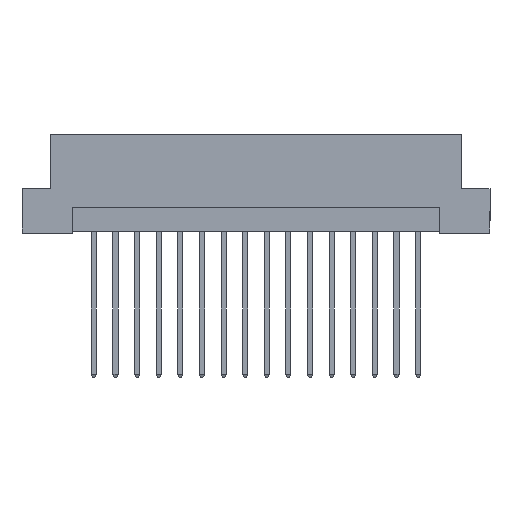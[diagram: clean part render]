
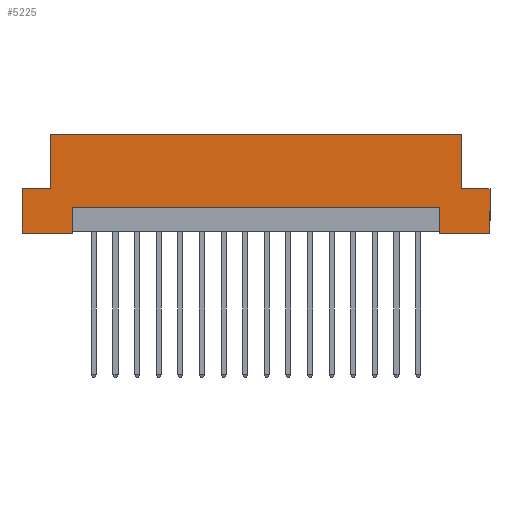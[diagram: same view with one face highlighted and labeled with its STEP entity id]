
A CAD part, front view. The second image highlights one B-rep face of the part: STEP entity #5225.
In plain terms, the highlighted planar face has unit normal (0, -1, 0).
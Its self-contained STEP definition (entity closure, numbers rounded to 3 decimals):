
#166 = ORIENTED_EDGE ( 'NONE', *, *, #7190, .F. ) ;
#254 = EDGE_CURVE ( 'NONE', #5056, #949, #5466, .T. ) ;
#280 = FACE_OUTER_BOUND ( 'NONE', #7388, .T. ) ;
#286 = CARTESIAN_POINT ( 'NONE',  ( 21.6, -4.3, 0.2 ) ) ;
#355 = DIRECTION ( 'NONE',  ( 1., 0., 0. ) ) ;
#407 = ORIENTED_EDGE ( 'NONE', *, *, #4334, .F. ) ;
#423 = EDGE_CURVE ( 'NONE', #5056, #5381, #3980, .T. ) ;
#424 = DIRECTION ( 'NONE',  ( 1., 0., 0. ) ) ;
#456 = CARTESIAN_POINT ( 'NONE',  ( -21.6, -4.3, 0.2 ) ) ;
#461 = DIRECTION ( 'NONE',  ( 1., 0., 0. ) ) ;
#501 = CARTESIAN_POINT ( 'NONE',  ( -24.2, -4.3, 11.6 ) ) ;
#583 = CARTESIAN_POINT ( 'NONE',  ( -27.5, -4.3, 5.2 ) ) ;
#593 = CARTESIAN_POINT ( 'NONE',  ( 21.6, -4.3, 3. ) ) ;
#705 = CARTESIAN_POINT ( 'NONE',  ( 27.5, -4.3, 11.6 ) ) ;
#861 = ORIENTED_EDGE ( 'NONE', *, *, #946, .F. ) ;
#903 = CARTESIAN_POINT ( 'NONE',  ( 24.2, -4.3, 5.2 ) ) ;
#932 = LINE ( 'NONE', #286, #4435 ) ;
#946 = EDGE_CURVE ( 'NONE', #5382, #5692, #3523, .T. ) ;
#949 = VERTEX_POINT ( 'NONE', #593 ) ;
#1036 = VECTOR ( 'NONE', #1269, 1000. ) ;
#1092 = ORIENTED_EDGE ( 'NONE', *, *, #1218, .F. ) ;
#1218 = EDGE_CURVE ( 'NONE', #6092, #949, #932, .T. ) ;
#1231 = ORIENTED_EDGE ( 'NONE', *, *, #1559, .F. ) ;
#1269 = DIRECTION ( 'NONE',  ( 0., 0., -1. ) ) ;
#1309 = CARTESIAN_POINT ( 'NONE',  ( -24.2, -4.3, 5.2 ) ) ;
#1356 = AXIS2_PLACEMENT_3D ( 'NONE', #7204, #1496, #2031 ) ;
#1485 = CARTESIAN_POINT ( 'NONE',  ( -21.6, -4.3, 3. ) ) ;
#1496 = DIRECTION ( 'NONE',  ( 0., 1., 0. ) ) ;
#1499 = EDGE_CURVE ( 'NONE', #5257, #5357, #5399, .T. ) ;
#1559 = EDGE_CURVE ( 'NONE', #2888, #5382, #4757, .T. ) ;
#1643 = EDGE_CURVE ( 'NONE', #2181, #5692, #3835, .T. ) ;
#1853 = VECTOR ( 'NONE', #461, 1000. ) ;
#1952 = VECTOR ( 'NONE', #355, 1000. ) ;
#2028 = CARTESIAN_POINT ( 'NONE',  ( -24.2, -4.3, 5.2 ) ) ;
#2031 = DIRECTION ( 'NONE',  ( -1., 0., 0. ) ) ;
#2127 = CARTESIAN_POINT ( 'NONE',  ( 24.2, -4.3, 11.6 ) ) ;
#2181 = VERTEX_POINT ( 'NONE', #903 ) ;
#2311 = CARTESIAN_POINT ( 'NONE',  ( 27.5, -4.3, 5.2 ) ) ;
#2312 = DIRECTION ( 'NONE',  ( 0., 0., -1. ) ) ;
#2378 = DIRECTION ( 'NONE',  ( 1., 0., 0. ) ) ;
#2584 = CARTESIAN_POINT ( 'NONE',  ( 24.2, -4.3, 5.2 ) ) ;
#2594 = VECTOR ( 'NONE', #7379, 1000. ) ;
#2819 = CARTESIAN_POINT ( 'NONE',  ( -27.5, -4.3, 5.2 ) ) ;
#2888 = VERTEX_POINT ( 'NONE', #2028 ) ;
#2912 = EDGE_CURVE ( 'NONE', #5357, #5381, #4299, .T. ) ;
#2960 = EDGE_CURVE ( 'NONE', #6092, #7219, #5544, .T. ) ;
#3172 = VECTOR ( 'NONE', #424, 1000. ) ;
#3177 = VECTOR ( 'NONE', #2312, 1000. ) ;
#3294 = CARTESIAN_POINT ( 'NONE',  ( 21.6, -4.3, 0. ) ) ;
#3344 = VECTOR ( 'NONE', #2378, 1000. ) ;
#3491 = LINE ( 'NONE', #2311, #4880 ) ;
#3492 = ORIENTED_EDGE ( 'NONE', *, *, #5794, .F. ) ;
#3523 = LINE ( 'NONE', #705, #3344 ) ;
#3625 = DIRECTION ( 'NONE',  ( 0., 0., 1. ) ) ;
#3835 = LINE ( 'NONE', #2584, #4684 ) ;
#3954 = CARTESIAN_POINT ( 'NONE',  ( -21.6, -4.3, 0. ) ) ;
#3980 = LINE ( 'NONE', #456, #2594 ) ;
#4271 = DIRECTION ( 'NONE',  ( 0., 0., 1. ) ) ;
#4291 = VECTOR ( 'NONE', #6670, 1000. ) ;
#4299 = LINE ( 'NONE', #6715, #3172 ) ;
#4334 = EDGE_CURVE ( 'NONE', #2181, #5126, #3491, .T. ) ;
#4435 = VECTOR ( 'NONE', #4271, 1000. ) ;
#4684 = VECTOR ( 'NONE', #6142, 1000. ) ;
#4692 = ORIENTED_EDGE ( 'NONE', *, *, #1499, .T. ) ;
#4757 = LINE ( 'NONE', #1309, #7321 ) ;
#4801 = ORIENTED_EDGE ( 'NONE', *, *, #423, .F. ) ;
#4880 = VECTOR ( 'NONE', #5238, 1000. ) ;
#4920 = PLANE ( 'NONE',  #1356 ) ;
#5056 = VERTEX_POINT ( 'NONE', #6505 ) ;
#5099 = LINE ( 'NONE', #2819, #1853 ) ;
#5126 = VERTEX_POINT ( 'NONE', #5546 ) ;
#5185 = CARTESIAN_POINT ( 'NONE',  ( -27.5, -4.3, 0. ) ) ;
#5225 = ADVANCED_FACE ( 'NONE', ( #280 ), #4920, .F. ) ;
#5238 = DIRECTION ( 'NONE',  ( 1., 0., 0. ) ) ;
#5257 = VERTEX_POINT ( 'NONE', #583 ) ;
#5357 = VERTEX_POINT ( 'NONE', #5185 ) ;
#5381 = VERTEX_POINT ( 'NONE', #3954 ) ;
#5382 = VERTEX_POINT ( 'NONE', #501 ) ;
#5399 = LINE ( 'NONE', #7161, #1036 ) ;
#5466 = LINE ( 'NONE', #1485, #4291 ) ;
#5544 = LINE ( 'NONE', #6106, #1952 ) ;
#5546 = CARTESIAN_POINT ( 'NONE',  ( 27.5, -4.3, 5.2 ) ) ;
#5692 = VERTEX_POINT ( 'NONE', #2127 ) ;
#5794 = EDGE_CURVE ( 'NONE', #5126, #7219, #6434, .T. ) ;
#5872 = ORIENTED_EDGE ( 'NONE', *, *, #1643, .T. ) ;
#6024 = ORIENTED_EDGE ( 'NONE', *, *, #2960, .T. ) ;
#6092 = VERTEX_POINT ( 'NONE', #3294 ) ;
#6106 = CARTESIAN_POINT ( 'NONE',  ( 27.5, -4.3, 0. ) ) ;
#6142 = DIRECTION ( 'NONE',  ( 0., 0., 1. ) ) ;
#6346 = ORIENTED_EDGE ( 'NONE', *, *, #2912, .T. ) ;
#6434 = LINE ( 'NONE', #7456, #3177 ) ;
#6505 = CARTESIAN_POINT ( 'NONE',  ( -21.6, -4.3, 3. ) ) ;
#6670 = DIRECTION ( 'NONE',  ( 1., 0., 0. ) ) ;
#6688 = ORIENTED_EDGE ( 'NONE', *, *, #254, .T. ) ;
#6715 = CARTESIAN_POINT ( 'NONE',  ( 27.5, -4.3, 0. ) ) ;
#7161 = CARTESIAN_POINT ( 'NONE',  ( -27.5, -4.3, 11.6 ) ) ;
#7190 = EDGE_CURVE ( 'NONE', #5257, #2888, #5099, .T. ) ;
#7204 = CARTESIAN_POINT ( 'NONE',  ( 27.5, -4.3, 11.6 ) ) ;
#7219 = VERTEX_POINT ( 'NONE', #7387 ) ;
#7321 = VECTOR ( 'NONE', #3625, 1000. ) ;
#7379 = DIRECTION ( 'NONE',  ( 0., 0., -1. ) ) ;
#7387 = CARTESIAN_POINT ( 'NONE',  ( 27.5, -4.3, 0. ) ) ;
#7388 = EDGE_LOOP ( 'NONE', ( #6688, #1092, #6024, #3492, #407, #5872, #861, #1231, #166, #4692, #6346, #4801 ) ) ;
#7456 = CARTESIAN_POINT ( 'NONE',  ( 27.5, -4.3, 11.6 ) ) ;
